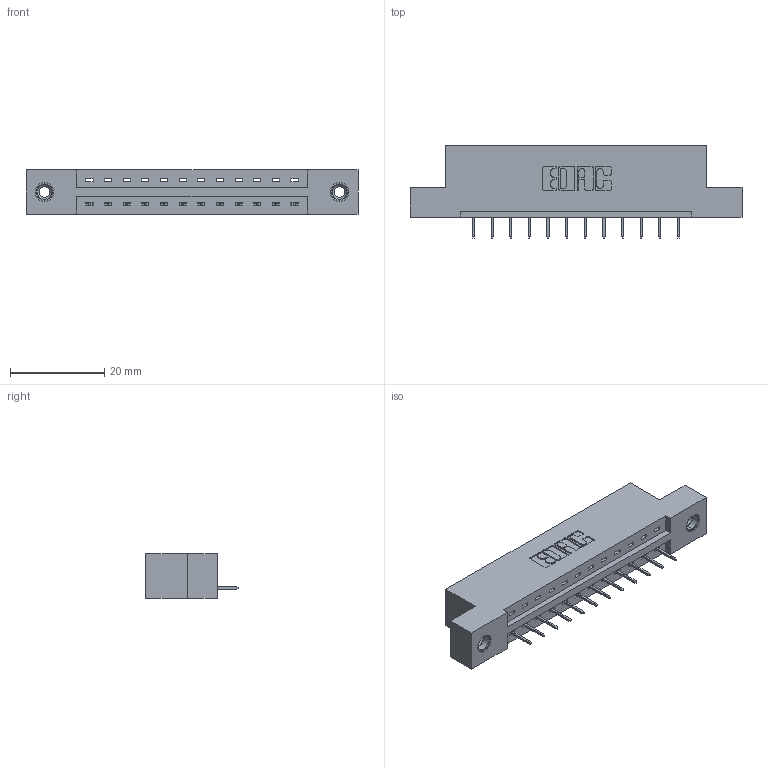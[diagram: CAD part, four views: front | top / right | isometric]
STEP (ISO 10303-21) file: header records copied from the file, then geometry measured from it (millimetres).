
FILE_DESCRIPTION (( 'STEP AP203' ), '1' );
FILE_NAME ('387-012-524-108.STEP', '2018-09-10T10:13:40', ( '' ), ( '' ), 'SwSTEP 2.0', 'SolidWorks 2016', '' );
FILE_SCHEMA (( 'CONFIG_CONTROL_DESIGN' ));
Length unit declared in the file: inch
Products named in the file (4): 387-012-524-108; 337 Part_Flush Mounting Lugs - 0.156 Dia-TI; 345-292-001_345-293-124; 345-250-001_345-250-003-102
Assembly tree (15 placements, depth 2):
  387-012-524-108
    337 Part_Flush Mounting Lugs - 0.156 Dia-TI
    345-292-001_345-293-124  x12
    345-250-001_345-250-003-102  x2
Bounding box: 70.56 x 19.69 x 9.4 mm (x, y, z)
Volume: 6904.3 mm3; surface area: 6831.1 mm2
Topology: 15 solids, 15 shells, 966 faces, 2751 edges, 1778 vertices
Faces by surface type: plane 726, cylinder 224, cone 12, torus 4
Entity records: 14060 total; most frequent: CARTESIAN_POINT 2425, ORIENTED_EDGE 2366, DIRECTION 2137, EDGE_CURVE 1183, LINE 1039, VECTOR 1039, VERTEX_POINT 780, AXIS2_PLACEMENT_3D 549
